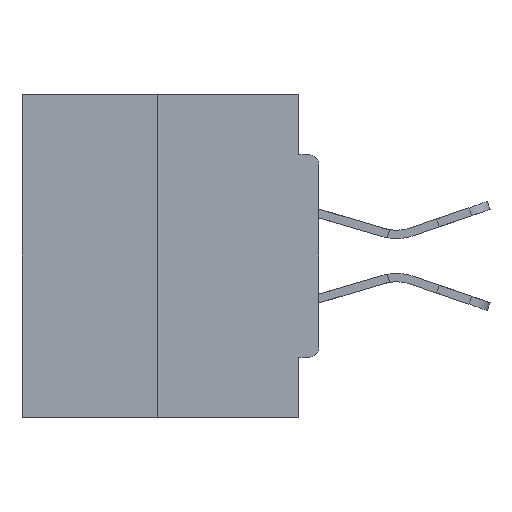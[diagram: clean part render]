
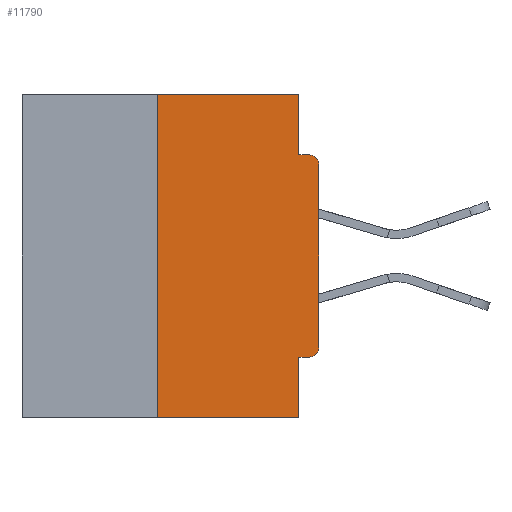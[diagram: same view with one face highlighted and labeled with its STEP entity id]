
A CAD part, left-side view. The second image highlights one B-rep face of the part: STEP entity #11790.
In plain terms, the highlighted planar face has unit normal (-1, 0, 0).
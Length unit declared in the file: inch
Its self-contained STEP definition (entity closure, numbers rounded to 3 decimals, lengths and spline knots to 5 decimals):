
#850 = CARTESIAN_POINT ( 'NONE',  ( 0., 0., -0.1085 ) ) ;
#1046 = CARTESIAN_POINT ( 'NONE',  ( 0., 0.031, 0. ) ) ;
#1153 = CARTESIAN_POINT ( 'NONE',  ( 0., 0.015, -0.0935 ) ) ;
#1269 = VERTEX_POINT ( 'NONE', #25700 ) ;
#1371 = LINE ( 'NONE', #27149, #5741 ) ;
#2099 = ORIENTED_EDGE ( 'NONE', *, *, #7736, .T. ) ;
#2101 = FACE_OUTER_BOUND ( 'NONE', #14584, .T. ) ;
#2189 = VECTOR ( 'NONE', #17362, 39.37008 ) ;
#2207 = LINE ( 'NONE', #1046, #15171 ) ;
#2900 = VECTOR ( 'NONE', #13166, 39.37008 ) ;
#3487 = VECTOR ( 'NONE', #5572, 39.37008 ) ;
#3615 = CARTESIAN_POINT ( 'NONE',  ( 0., 0.015, -0.1085 ) ) ;
#3652 = DIRECTION ( 'NONE',  ( 0., 0., 1. ) ) ;
#3860 = DIRECTION ( 'NONE',  ( 0., 0., -1. ) ) ;
#4099 = CARTESIAN_POINT ( 'NONE',  ( 0., 0.46, 0. ) ) ;
#4294 = DIRECTION ( 'NONE',  ( 1., 0., 0. ) ) ;
#4432 = ORIENTED_EDGE ( 'NONE', *, *, #34818, .F. ) ;
#5138 = VERTEX_POINT ( 'NONE', #24914 ) ;
#5318 = VERTEX_POINT ( 'NONE', #8877 ) ;
#5572 = DIRECTION ( 'NONE',  ( 0., -1., 0. ) ) ;
#5741 = VECTOR ( 'NONE', #13253, 39.37008 ) ;
#6166 = CARTESIAN_POINT ( 'NONE',  ( 0., 0.015, -0.3915 ) ) ;
#6397 = DIRECTION ( 'NONE',  ( -1., 0., 0. ) ) ;
#7287 = VERTEX_POINT ( 'NONE', #17466 ) ;
#7484 = AXIS2_PLACEMENT_3D ( 'NONE', #3615, #6397, #19893 ) ;
#7736 = EDGE_CURVE ( 'NONE', #14598, #31167, #11094, .T. ) ;
#8333 = CARTESIAN_POINT ( 'NONE',  ( 0., 0.031, -0.0935 ) ) ;
#8877 = CARTESIAN_POINT ( 'NONE',  ( 0., 0.031, 0. ) ) ;
#8891 = ORIENTED_EDGE ( 'NONE', *, *, #29549, .F. ) ;
#10263 = LINE ( 'NONE', #24388, #2900 ) ;
#11094 = CIRCLE ( 'NONE', #7484, 0.015 ) ;
#11147 = CARTESIAN_POINT ( 'NONE',  ( 0., 0.015, -0.4065 ) ) ;
#11229 = EDGE_CURVE ( 'NONE', #31630, #7287, #35411, .T. ) ;
#11790 = ADVANCED_FACE ( 'NONE', ( #2101 ), #12351, .F. ) ;
#12351 = PLANE ( 'NONE',  #33917 ) ;
#13166 = DIRECTION ( 'NONE',  ( 0., 1., 0. ) ) ;
#13253 = DIRECTION ( 'NONE',  ( 0., 0., -1. ) ) ;
#13687 = LINE ( 'NONE', #24597, #17141 ) ;
#14149 = AXIS2_PLACEMENT_3D ( 'NONE', #6166, #19776, #33556 ) ;
#14584 = EDGE_LOOP ( 'NONE', ( #30788, #8891, #28163, #21009, #4432, #30492, #30934, #2099, #34863, #17016 ) ) ;
#14598 = VERTEX_POINT ( 'NONE', #850 ) ;
#14616 = DIRECTION ( 'NONE',  ( 0., 0., 1. ) ) ;
#15171 = VECTOR ( 'NONE', #3860, 39.37008 ) ;
#15251 = CARTESIAN_POINT ( 'NONE',  ( 0., 0.46, 0. ) ) ;
#15260 = VECTOR ( 'NONE', #14616, 39.37008 ) ;
#15965 = VERTEX_POINT ( 'NONE', #17595 ) ;
#16491 = CARTESIAN_POINT ( 'NONE',  ( 0., 0.46, -0.5 ) ) ;
#16780 = CARTESIAN_POINT ( 'NONE',  ( 0., 0.25, 0. ) ) ;
#17016 = ORIENTED_EDGE ( 'NONE', *, *, #22432, .F. ) ;
#17141 = VECTOR ( 'NONE', #32696, 39.37008 ) ;
#17362 = DIRECTION ( 'NONE',  ( 0., -1., 0. ) ) ;
#17466 = CARTESIAN_POINT ( 'NONE',  ( 0., 0.031, -0.5 ) ) ;
#17595 = CARTESIAN_POINT ( 'NONE',  ( 0., 0., -0.3915 ) ) ;
#18161 = EDGE_CURVE ( 'NONE', #5138, #7287, #1371, .T. ) ;
#19051 = EDGE_CURVE ( 'NONE', #15965, #14598, #23070, .T. ) ;
#19776 = DIRECTION ( 'NONE',  ( -1., 0., 0. ) ) ;
#19893 = DIRECTION ( 'NONE',  ( 0., 0., -1. ) ) ;
#21009 = ORIENTED_EDGE ( 'NONE', *, *, #18161, .F. ) ;
#21322 = LINE ( 'NONE', #16780, #15260 ) ;
#22432 = EDGE_CURVE ( 'NONE', #5318, #34947, #2207, .T. ) ;
#22442 = CIRCLE ( 'NONE', #14149, 0.015 ) ;
#23070 = LINE ( 'NONE', #33696, #28674 ) ;
#24388 = CARTESIAN_POINT ( 'NONE',  ( 0., 0., -0.4065 ) ) ;
#24597 = CARTESIAN_POINT ( 'NONE',  ( 0., 0., -0.0935 ) ) ;
#24914 = CARTESIAN_POINT ( 'NONE',  ( 0., 0.031, -0.4065 ) ) ;
#25700 = CARTESIAN_POINT ( 'NONE',  ( 0., 0.25, 0. ) ) ;
#26849 = LINE ( 'NONE', #4099, #2189 ) ;
#26940 = EDGE_CURVE ( 'NONE', #34947, #31167, #13687, .T. ) ;
#27149 = CARTESIAN_POINT ( 'NONE',  ( 0., 0.031, -0.5 ) ) ;
#28163 = ORIENTED_EDGE ( 'NONE', *, *, #11229, .T. ) ;
#28674 = VECTOR ( 'NONE', #3652, 39.37008 ) ;
#29549 = EDGE_CURVE ( 'NONE', #31630, #1269, #21322, .T. ) ;
#30492 = ORIENTED_EDGE ( 'NONE', *, *, #31637, .T. ) ;
#30623 = VERTEX_POINT ( 'NONE', #11147 ) ;
#30788 = ORIENTED_EDGE ( 'NONE', *, *, #32372, .F. ) ;
#30934 = ORIENTED_EDGE ( 'NONE', *, *, #19051, .T. ) ;
#31167 = VERTEX_POINT ( 'NONE', #1153 ) ;
#31630 = VERTEX_POINT ( 'NONE', #35351 ) ;
#31637 = EDGE_CURVE ( 'NONE', #30623, #15965, #22442, .T. ) ;
#31666 = DIRECTION ( 'NONE',  ( 0., 0., -1. ) ) ;
#32372 = EDGE_CURVE ( 'NONE', #1269, #5318, #26849, .T. ) ;
#32696 = DIRECTION ( 'NONE',  ( 0., -1., 0. ) ) ;
#33556 = DIRECTION ( 'NONE',  ( 0., 0., -1. ) ) ;
#33696 = CARTESIAN_POINT ( 'NONE',  ( 0., 0., 0. ) ) ;
#33917 = AXIS2_PLACEMENT_3D ( 'NONE', #15251, #4294, #31666 ) ;
#34818 = EDGE_CURVE ( 'NONE', #30623, #5138, #10263, .T. ) ;
#34863 = ORIENTED_EDGE ( 'NONE', *, *, #26940, .F. ) ;
#34947 = VERTEX_POINT ( 'NONE', #8333 ) ;
#35351 = CARTESIAN_POINT ( 'NONE',  ( 0., 0.25, -0.5 ) ) ;
#35411 = LINE ( 'NONE', #16491, #3487 ) ;
